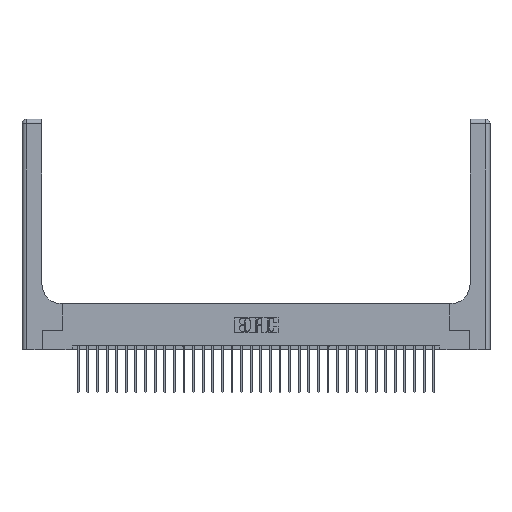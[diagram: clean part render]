
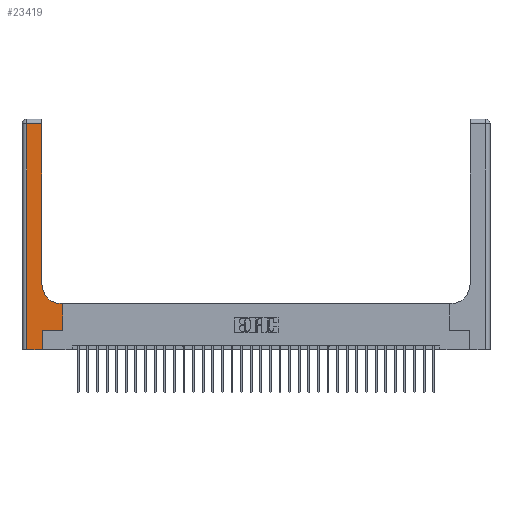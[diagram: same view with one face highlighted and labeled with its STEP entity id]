
A CAD part, top view. The second image highlights one B-rep face of the part: STEP entity #23419.
In plain terms, the highlighted planar face has unit normal (0, 0, 1).
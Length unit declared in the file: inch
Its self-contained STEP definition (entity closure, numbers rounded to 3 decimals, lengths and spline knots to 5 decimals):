
#82 = VERTEX_POINT ( 'NONE', #16807 ) ;
#300 = DIRECTION ( 'NONE',  ( 1., 0., 0. ) ) ;
#383 = CARTESIAN_POINT ( 'NONE',  ( 0.26, 2.94, 0.37 ) ) ;
#849 = LINE ( 'NONE', #24850, #26593 ) ;
#869 = ORIENTED_EDGE ( 'NONE', *, *, #27062, .T. ) ;
#2401 = DIRECTION ( 'NONE',  ( -1., 0., 0. ) ) ;
#3074 = VECTOR ( 'NONE', #29072, 39.37008 ) ;
#4458 = CARTESIAN_POINT ( 'NONE',  ( 0.26, 0.6, 0.37 ) ) ;
#4880 = DIRECTION ( 'NONE',  ( 0., 0., -1. ) ) ;
#5163 = CARTESIAN_POINT ( 'NONE',  ( 0.265, 0.25, 0.37 ) ) ;
#5339 = VERTEX_POINT ( 'NONE', #7835 ) ;
#5560 = VECTOR ( 'NONE', #15401, 39.37008 ) ;
#5758 = EDGE_CURVE ( 'NONE', #82, #9672, #849, .T. ) ;
#5990 = CARTESIAN_POINT ( 'NONE',  ( 0.265, 0., 0.37 ) ) ;
#6447 = AXIS2_PLACEMENT_3D ( 'NONE', #17209, #4880, #15022 ) ;
#6595 = CARTESIAN_POINT ( 'NONE',  ( 0.528, 0.25, 0.37 ) ) ;
#6732 = CARTESIAN_POINT ( 'NONE',  ( 0.51, 0.6, 0.37 ) ) ;
#7799 = CARTESIAN_POINT ( 'NONE',  ( 0., 2.94, 0.37 ) ) ;
#7835 = CARTESIAN_POINT ( 'NONE',  ( 0.528, 0.6, 0.37 ) ) ;
#7838 = DIRECTION ( 'NONE',  ( -1., 0., 0. ) ) ;
#7926 = ORIENTED_EDGE ( 'NONE', *, *, #12042, .T. ) ;
#7934 = ORIENTED_EDGE ( 'NONE', *, *, #16720, .T. ) ;
#8089 = ORIENTED_EDGE ( 'NONE', *, *, #12319, .T. ) ;
#8314 = DIRECTION ( 'NONE',  ( 0., 1., 0. ) ) ;
#8809 = DIRECTION ( 'NONE',  ( 0., -1., 0. ) ) ;
#9672 = VERTEX_POINT ( 'NONE', #26647 ) ;
#10148 = VECTOR ( 'NONE', #8809, 39.37008 ) ;
#10411 = ORIENTED_EDGE ( 'NONE', *, *, #12558, .T. ) ;
#10416 = CARTESIAN_POINT ( 'NONE',  ( 0.06, 2.94, 0.37 ) ) ;
#10476 = VERTEX_POINT ( 'NONE', #383 ) ;
#11328 = LINE ( 'NONE', #4458, #27983 ) ;
#12042 = EDGE_CURVE ( 'NONE', #5339, #28698, #11328, .T. ) ;
#12319 = EDGE_CURVE ( 'NONE', #25400, #10476, #20088, .T. ) ;
#12510 = EDGE_CURVE ( 'NONE', #14783, #19514, #21802, .T. ) ;
#12558 = EDGE_CURVE ( 'NONE', #28698, #25400, #19981, .T. ) ;
#13666 = CARTESIAN_POINT ( 'NONE',  ( 0.06, 3., 0.37 ) ) ;
#14335 = CARTESIAN_POINT ( 'NONE',  ( 0.528, 0.25, 0.37 ) ) ;
#14783 = VERTEX_POINT ( 'NONE', #18691 ) ;
#15022 = DIRECTION ( 'NONE',  ( 1., 0., 0. ) ) ;
#15319 = LINE ( 'NONE', #7799, #15692 ) ;
#15401 = DIRECTION ( 'NONE',  ( 0., 1., 0. ) ) ;
#15692 = VECTOR ( 'NONE', #27566, 39.37008 ) ;
#15953 = VECTOR ( 'NONE', #300, 39.37008 ) ;
#16720 = EDGE_CURVE ( 'NONE', #9672, #14783, #27341, .T. ) ;
#16807 = CARTESIAN_POINT ( 'NONE',  ( 0.06, 0., 0.37 ) ) ;
#17209 = CARTESIAN_POINT ( 'NONE',  ( 0.51, 0.85, 0.37 ) ) ;
#17469 = DIRECTION ( 'NONE',  ( 1., 0., 0. ) ) ;
#17658 = EDGE_LOOP ( 'NONE', ( #8089, #30329, #20373, #18944, #7934, #26930, #869, #7926, #10411 ) ) ;
#18691 = CARTESIAN_POINT ( 'NONE',  ( 0.265, 0.25, 0.37 ) ) ;
#18940 = CARTESIAN_POINT ( 'NONE',  ( 0.26, 0.85, 0.37 ) ) ;
#18944 = ORIENTED_EDGE ( 'NONE', *, *, #5758, .T. ) ;
#19310 = CARTESIAN_POINT ( 'NONE',  ( 0., 3., 0.37 ) ) ;
#19360 = LINE ( 'NONE', #14335, #3074 ) ;
#19454 = DIRECTION ( 'NONE',  ( 0., 0., -1. ) ) ;
#19514 = VERTEX_POINT ( 'NONE', #6595 ) ;
#19981 = CIRCLE ( 'NONE', #6447, 0.25 ) ;
#20088 = LINE ( 'NONE', #22602, #20986 ) ;
#20373 = ORIENTED_EDGE ( 'NONE', *, *, #28193, .T. ) ;
#20986 = VECTOR ( 'NONE', #8314, 39.37008 ) ;
#21663 = FACE_OUTER_BOUND ( 'NONE', #17658, .T. ) ;
#21802 = LINE ( 'NONE', #5163, #15953 ) ;
#22602 = CARTESIAN_POINT ( 'NONE',  ( 0.26, 3., 0.37 ) ) ;
#22827 = EDGE_CURVE ( 'NONE', #10476, #29318, #15319, .T. ) ;
#23419 = ADVANCED_FACE ( 'NONE', ( #21663 ), #24318, .F. ) ;
#24318 = PLANE ( 'NONE',  #24787 ) ;
#24787 = AXIS2_PLACEMENT_3D ( 'NONE', #19310, #19454, #7838 ) ;
#24850 = CARTESIAN_POINT ( 'NONE',  ( 0., 0., 0.37 ) ) ;
#25400 = VERTEX_POINT ( 'NONE', #18940 ) ;
#26593 = VECTOR ( 'NONE', #17469, 39.37008 ) ;
#26647 = CARTESIAN_POINT ( 'NONE',  ( 0.265, 0., 0.37 ) ) ;
#26930 = ORIENTED_EDGE ( 'NONE', *, *, #12510, .T. ) ;
#27062 = EDGE_CURVE ( 'NONE', #19514, #5339, #19360, .T. ) ;
#27341 = LINE ( 'NONE', #5990, #5560 ) ;
#27566 = DIRECTION ( 'NONE',  ( -1., 0., 0. ) ) ;
#27983 = VECTOR ( 'NONE', #2401, 39.37008 ) ;
#28193 = EDGE_CURVE ( 'NONE', #29318, #82, #30306, .T. ) ;
#28698 = VERTEX_POINT ( 'NONE', #6732 ) ;
#29072 = DIRECTION ( 'NONE',  ( 0., 1., 0. ) ) ;
#29318 = VERTEX_POINT ( 'NONE', #10416 ) ;
#30306 = LINE ( 'NONE', #13666, #10148 ) ;
#30329 = ORIENTED_EDGE ( 'NONE', *, *, #22827, .T. ) ;
